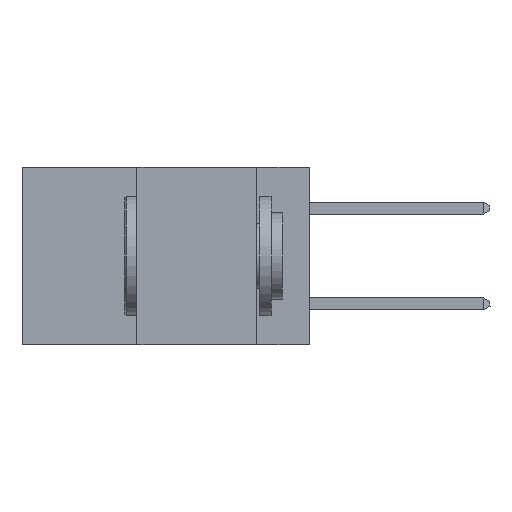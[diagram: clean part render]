
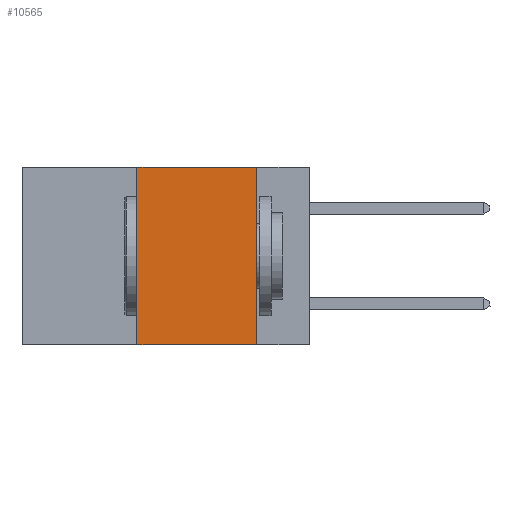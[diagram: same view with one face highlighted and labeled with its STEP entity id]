
A CAD part, left-side view. The second image highlights one B-rep face of the part: STEP entity #10565.
In plain terms, the highlighted planar face has unit normal (-1, 0, 0).
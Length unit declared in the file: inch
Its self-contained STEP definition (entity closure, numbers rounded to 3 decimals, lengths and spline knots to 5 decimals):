
#190 = DIRECTION ( 'NONE',  ( 0., 0., 1. ) ) ;
#729 = DIRECTION ( 'NONE',  ( 0., 0., -1. ) ) ;
#1220 = AXIS2_PLACEMENT_3D ( 'NONE', #9548, #11247, #729 ) ;
#1615 = VECTOR ( 'NONE', #16891, 39.37008 ) ;
#2180 = LINE ( 'NONE', #21961, #1615 ) ;
#2910 = LINE ( 'NONE', #3217, #20857 ) ;
#3217 = CARTESIAN_POINT ( 'NONE',  ( 0., 0.6, -0.37 ) ) ;
#3765 = EDGE_LOOP ( 'NONE', ( #6895, #11673, #9815, #3845 ) ) ;
#3845 = ORIENTED_EDGE ( 'NONE', *, *, #5492, .T. ) ;
#3858 = CARTESIAN_POINT ( 'NONE',  ( 0., 0.36, 0. ) ) ;
#5492 = EDGE_CURVE ( 'NONE', #12196, #7480, #2910, .T. ) ;
#5707 = CARTESIAN_POINT ( 'NONE',  ( 0., 0.36, -0.37 ) ) ;
#6862 = CARTESIAN_POINT ( 'NONE',  ( 0., 0.6, 0. ) ) ;
#6895 = ORIENTED_EDGE ( 'NONE', *, *, #17406, .F. ) ;
#7480 = VERTEX_POINT ( 'NONE', #12957 ) ;
#8180 = VECTOR ( 'NONE', #8552, 39.37008 ) ;
#8552 = DIRECTION ( 'NONE',  ( 0., -1., 0. ) ) ;
#8883 = VERTEX_POINT ( 'NONE', #11955 ) ;
#9548 = CARTESIAN_POINT ( 'NONE',  ( 0., 0.6, 0. ) ) ;
#9815 = ORIENTED_EDGE ( 'NONE', *, *, #19272, .F. ) ;
#10003 = FACE_OUTER_BOUND ( 'NONE', #3765, .T. ) ;
#10565 = ADVANCED_FACE ( 'NONE', ( #10003 ), #19941, .F. ) ;
#11247 = DIRECTION ( 'NONE',  ( 1., 0., 0. ) ) ;
#11673 = ORIENTED_EDGE ( 'NONE', *, *, #20343, .F. ) ;
#11955 = CARTESIAN_POINT ( 'NONE',  ( 0., 0.36, 0. ) ) ;
#12196 = VERTEX_POINT ( 'NONE', #5707 ) ;
#12526 = LINE ( 'NONE', #3858, #17193 ) ;
#12760 = LINE ( 'NONE', #6862, #8180 ) ;
#12957 = CARTESIAN_POINT ( 'NONE',  ( 0., 0.11, -0.37 ) ) ;
#13010 = VERTEX_POINT ( 'NONE', #16352 ) ;
#16352 = CARTESIAN_POINT ( 'NONE',  ( 0., 0.11, 0. ) ) ;
#16891 = DIRECTION ( 'NONE',  ( 0., 0., -1. ) ) ;
#17193 = VECTOR ( 'NONE', #190, 39.37008 ) ;
#17406 = EDGE_CURVE ( 'NONE', #13010, #7480, #2180, .T. ) ;
#19272 = EDGE_CURVE ( 'NONE', #12196, #8883, #12526, .T. ) ;
#19941 = PLANE ( 'NONE',  #1220 ) ;
#20343 = EDGE_CURVE ( 'NONE', #8883, #13010, #12760, .T. ) ;
#20609 = DIRECTION ( 'NONE',  ( 0., -1., 0. ) ) ;
#20857 = VECTOR ( 'NONE', #20609, 39.37008 ) ;
#21961 = CARTESIAN_POINT ( 'NONE',  ( 0., 0.11, 0. ) ) ;
